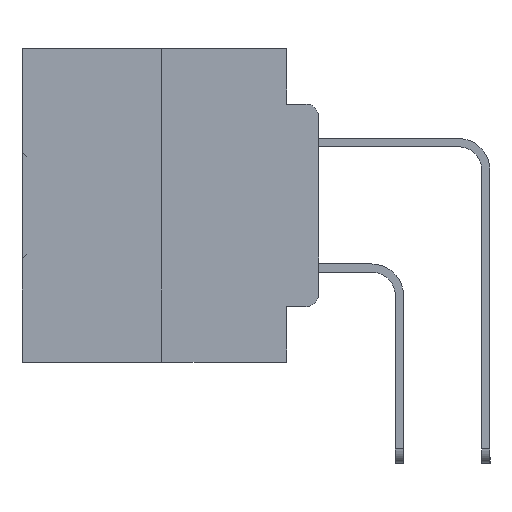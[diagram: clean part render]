
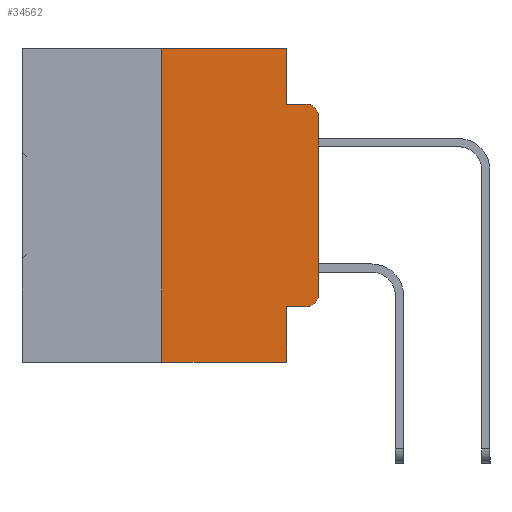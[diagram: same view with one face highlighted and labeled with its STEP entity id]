
A CAD part, left-side view. The second image highlights one B-rep face of the part: STEP entity #34562.
In plain terms, the highlighted planar face has unit normal (-1, 0, 0).
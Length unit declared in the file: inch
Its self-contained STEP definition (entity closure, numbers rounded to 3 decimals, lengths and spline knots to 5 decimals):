
#314 = ORIENTED_EDGE ( 'NONE', *, *, #13798, .T. ) ;
#1226 = VERTEX_POINT ( 'NONE', #23754 ) ;
#1387 = DIRECTION ( 'NONE',  ( 1., 0., 0. ) ) ;
#1803 = VERTEX_POINT ( 'NONE', #36399 ) ;
#1972 = VERTEX_POINT ( 'NONE', #33616 ) ;
#2742 = VECTOR ( 'NONE', #5648, 39.37008 ) ;
#3416 = CARTESIAN_POINT ( 'NONE',  ( 0., 0.051, -0.4115 ) ) ;
#3459 = ORIENTED_EDGE ( 'NONE', *, *, #5635, .F. ) ;
#3710 = EDGE_CURVE ( 'NONE', #4539, #24008, #21610, .T. ) ;
#4539 = VERTEX_POINT ( 'NONE', #19771 ) ;
#5119 = LINE ( 'NONE', #32578, #12735 ) ;
#5635 = EDGE_CURVE ( 'NONE', #24008, #1226, #22245, .T. ) ;
#5648 = DIRECTION ( 'NONE',  ( 0., 0., -1. ) ) ;
#6326 = DIRECTION ( 'NONE',  ( 0., -1., 0. ) ) ;
#6679 = VECTOR ( 'NONE', #32511, 39.37008 ) ;
#7165 = VECTOR ( 'NONE', #9610, 39.37008 ) ;
#7197 = CARTESIAN_POINT ( 'NONE',  ( 0., 0.25, 0. ) ) ;
#7576 = EDGE_LOOP ( 'NONE', ( #14207, #23467, #3459, #33422, #35157, #13772, #314, #15573, #23050, #32168 ) ) ;
#7583 = EDGE_CURVE ( 'NONE', #33326, #1226, #21247, .T. ) ;
#7984 = VERTEX_POINT ( 'NONE', #9202 ) ;
#9202 = CARTESIAN_POINT ( 'NONE',  ( 0., 0., -0.3915 ) ) ;
#9316 = CARTESIAN_POINT ( 'NONE',  ( 0., 0.051, -0.0885 ) ) ;
#9546 = VERTEX_POINT ( 'NONE', #22915 ) ;
#9610 = DIRECTION ( 'NONE',  ( 0., -1., 0. ) ) ;
#10217 = CARTESIAN_POINT ( 'NONE',  ( 0., 0.02, -0.1085 ) ) ;
#10374 = DIRECTION ( 'NONE',  ( 0., -1., 0. ) ) ;
#10503 = CARTESIAN_POINT ( 'NONE',  ( 0., 0.473, 0. ) ) ;
#10975 = LINE ( 'NONE', #10503, #26803 ) ;
#11276 = CARTESIAN_POINT ( 'NONE',  ( 0., 0.051, 0. ) ) ;
#11968 = VECTOR ( 'NONE', #6326, 39.37008 ) ;
#12570 = DIRECTION ( 'NONE',  ( -1., 0., 0. ) ) ;
#12735 = VECTOR ( 'NONE', #32467, 39.37008 ) ;
#13064 = DIRECTION ( 'NONE',  ( 0., 0., -1. ) ) ;
#13304 = EDGE_CURVE ( 'NONE', #7984, #33326, #27696, .T. ) ;
#13644 = DIRECTION ( 'NONE',  ( 0., 0., -1. ) ) ;
#13772 = ORIENTED_EDGE ( 'NONE', *, *, #34581, .F. ) ;
#13798 = EDGE_CURVE ( 'NONE', #9546, #23575, #5119, .T. ) ;
#14207 = ORIENTED_EDGE ( 'NONE', *, *, #13304, .T. ) ;
#14499 = CARTESIAN_POINT ( 'NONE',  ( 0., 0., -0.1085 ) ) ;
#15166 = FACE_OUTER_BOUND ( 'NONE', #7576, .T. ) ;
#15573 = ORIENTED_EDGE ( 'NONE', *, *, #32747, .F. ) ;
#15672 = PLANE ( 'NONE',  #35658 ) ;
#15787 = CARTESIAN_POINT ( 'NONE',  ( 0., 0.25, 0. ) ) ;
#16044 = CIRCLE ( 'NONE', #16956, 0.02 ) ;
#16956 = AXIS2_PLACEMENT_3D ( 'NONE', #29383, #12570, #32160 ) ;
#19481 = CARTESIAN_POINT ( 'NONE',  ( 0., 0., 0. ) ) ;
#19771 = CARTESIAN_POINT ( 'NONE',  ( 0., 0.051, 0. ) ) ;
#20293 = VECTOR ( 'NONE', #36102, 39.37008 ) ;
#21247 = CIRCLE ( 'NONE', #27134, 0.02 ) ;
#21349 = DIRECTION ( 'NONE',  ( 0., 0., -1. ) ) ;
#21476 = CARTESIAN_POINT ( 'NONE',  ( 0., 0.051, -0.5 ) ) ;
#21610 = LINE ( 'NONE', #11276, #35462 ) ;
#22245 = LINE ( 'NONE', #32040, #7165 ) ;
#22915 = CARTESIAN_POINT ( 'NONE',  ( 0., 0.25, -0.5 ) ) ;
#23038 = EDGE_CURVE ( 'NONE', #23564, #4539, #10975, .T. ) ;
#23050 = ORIENTED_EDGE ( 'NONE', *, *, #25319, .T. ) ;
#23465 = EDGE_CURVE ( 'NONE', #1972, #7984, #16044, .T. ) ;
#23467 = ORIENTED_EDGE ( 'NONE', *, *, #7583, .T. ) ;
#23564 = VERTEX_POINT ( 'NONE', #15787 ) ;
#23575 = VERTEX_POINT ( 'NONE', #21476 ) ;
#23754 = CARTESIAN_POINT ( 'NONE',  ( 0., 0.02, -0.0885 ) ) ;
#24008 = VERTEX_POINT ( 'NONE', #9316 ) ;
#25319 = EDGE_CURVE ( 'NONE', #1803, #1972, #34248, .T. ) ;
#26803 = VECTOR ( 'NONE', #10374, 39.37008 ) ;
#27134 = AXIS2_PLACEMENT_3D ( 'NONE', #10217, #29862, #13064 ) ;
#27696 = LINE ( 'NONE', #19481, #20293 ) ;
#29165 = LINE ( 'NONE', #7197, #6679 ) ;
#29383 = CARTESIAN_POINT ( 'NONE',  ( 0., 0.02, -0.3915 ) ) ;
#29862 = DIRECTION ( 'NONE',  ( -1., 0., 0. ) ) ;
#31883 = LINE ( 'NONE', #33783, #2742 ) ;
#32040 = CARTESIAN_POINT ( 'NONE',  ( 0., 0.051, -0.0885 ) ) ;
#32160 = DIRECTION ( 'NONE',  ( 0., 0., -1. ) ) ;
#32168 = ORIENTED_EDGE ( 'NONE', *, *, #23465, .T. ) ;
#32467 = DIRECTION ( 'NONE',  ( 0., -1., 0. ) ) ;
#32511 = DIRECTION ( 'NONE',  ( 0., 0., 1. ) ) ;
#32578 = CARTESIAN_POINT ( 'NONE',  ( 0., 0.473, -0.5 ) ) ;
#32747 = EDGE_CURVE ( 'NONE', #1803, #23575, #31883, .T. ) ;
#33326 = VERTEX_POINT ( 'NONE', #14499 ) ;
#33422 = ORIENTED_EDGE ( 'NONE', *, *, #3710, .F. ) ;
#33616 = CARTESIAN_POINT ( 'NONE',  ( 0., 0.02, -0.4115 ) ) ;
#33783 = CARTESIAN_POINT ( 'NONE',  ( 0., 0.051, 0. ) ) ;
#34248 = LINE ( 'NONE', #3416, #11968 ) ;
#34562 = ADVANCED_FACE ( 'NONE', ( #15166 ), #15672, .F. ) ;
#34581 = EDGE_CURVE ( 'NONE', #9546, #23564, #29165, .T. ) ;
#35148 = CARTESIAN_POINT ( 'NONE',  ( 0., 0.473, 0. ) ) ;
#35157 = ORIENTED_EDGE ( 'NONE', *, *, #23038, .F. ) ;
#35462 = VECTOR ( 'NONE', #13644, 39.37008 ) ;
#35658 = AXIS2_PLACEMENT_3D ( 'NONE', #35148, #1387, #21349 ) ;
#36102 = DIRECTION ( 'NONE',  ( 0., 0., 1. ) ) ;
#36399 = CARTESIAN_POINT ( 'NONE',  ( 0., 0.051, -0.4115 ) ) ;
